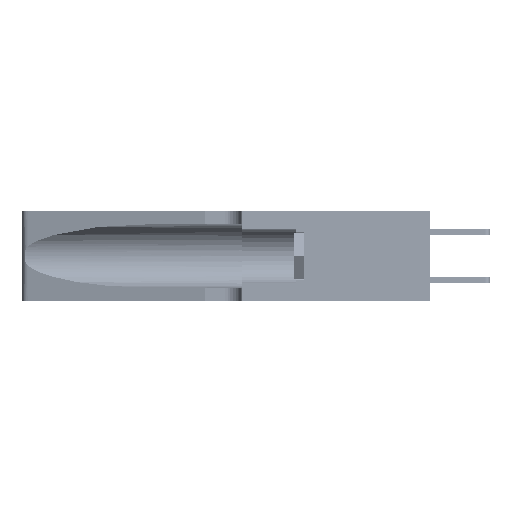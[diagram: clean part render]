
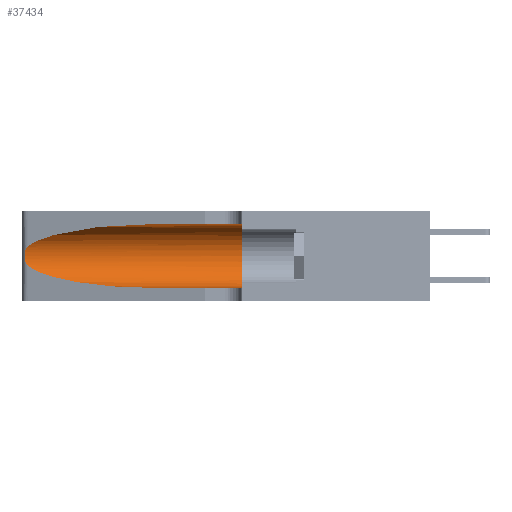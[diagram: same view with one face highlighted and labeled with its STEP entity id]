
A CAD part, left-side view. The second image highlights one B-rep face of the part: STEP entity #37434.
In plain terms, the highlighted cylindrical face has radius 3.308 mm (diameter 6.617 mm), a partial arc.
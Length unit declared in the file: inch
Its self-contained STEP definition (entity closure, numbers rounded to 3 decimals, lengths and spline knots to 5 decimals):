
#16 = ORIENTED_EDGE ( 'NONE', *, *, #25882, .T. ) ;
#394 = CARTESIAN_POINT ( 'NONE',  ( 0.26018, 1.23835, 0.19895 ) ) ;
#537 = CARTESIAN_POINT ( 'NONE',  ( 0.26017, 1.23833, 0.17102 ) ) ;
#4063 = CARTESIAN_POINT ( 'NONE',  ( 0.26075, 1.23896, 0.19203 ) ) ;
#4191 = CARTESIAN_POINT ( 'NONE',  ( 0.25856, 1.23593, 0.16098 ) ) ;
#4660 = DIRECTION ( 'NONE',  ( 0., -1., 0. ) ) ;
#5260 = FACE_OUTER_BOUND ( 'NONE', #7107, .T. ) ;
#5830 = LINE ( 'NONE', #11191, #22958 ) ;
#7107 = EDGE_LOOP ( 'NONE', ( #22844, #28178, #16, #17809, #18343, #36347 ) ) ;
#7213 = EDGE_CURVE ( 'NONE', #29267, #22690, #15760, .T. ) ;
#7237 = CARTESIAN_POINT ( 'NONE',  ( 0.25487, 1.22718, 0.14631 ) ) ;
#7265 = CYLINDRICAL_SURFACE ( 'NONE', #29936, 0.13025 ) ;
#7520 = CARTESIAN_POINT ( 'NONE',  ( 0.25787, 1.23484, 0.2124 ) ) ;
#7990 = CARTESIAN_POINT ( 'NONE',  ( 0.1305, 1.61858, 0.185 ) ) ;
#8094 = CARTESIAN_POINT ( 'NONE',  ( 0.1305, 0.72297, 0.05475 ) ) ;
#8631 = EDGE_CURVE ( 'NONE', #36880, #33583, #22777, .T. ) ;
#8737 = DIRECTION ( 'NONE',  ( 0., 0., 1. ) ) ;
#9618 = VECTOR ( 'NONE', #12274, 39.37008 ) ;
#11191 = CARTESIAN_POINT ( 'NONE',  ( 0.1305, 1.61858, 0.05475 ) ) ;
#11866 = VERTEX_POINT ( 'NONE', #37948 ) ;
#12274 = DIRECTION ( 'NONE',  ( 0., -1., 0. ) ) ;
#13554 = CARTESIAN_POINT ( 'NONE',  ( 0.1305, 0.35, 0.05475 ) ) ;
#15760 =( BOUNDED_CURVE ( )  B_SPLINE_CURVE ( 3, ( #37120, #20581, #34031, #32048 ),
 .UNSPECIFIED., .F., .F. ) 
 B_SPLINE_CURVE_WITH_KNOTS ( ( 4, 4 ),
 ( 1.5708, 2.84003 ),
 .UNSPECIFIED. ) 
 CURVE ( )  GEOMETRIC_REPRESENTATION_ITEM ( )  RATIONAL_B_SPLINE_CURVE ( ( 1., 0.87, 0.87, 1. ) ) 
 REPRESENTATION_ITEM ( '' )  );
#17014 = B_SPLINE_CURVE_WITH_KNOTS ( 'NONE', 3,
 ( #24036, #36865, #20741, #7520, #37137, #394, #4063, #20328, #537, #4191, #27388, #30696, #40222, #7237 ),
 .UNSPECIFIED., .F., .F.,
 ( 4, 2, 2, 2, 2, 2, 4 ),
 ( 0., 0.00027, 0.00053, 0.00107, 0.0016, 0.00187, 0.00214 ),
 .UNSPECIFIED. ) ;
#17809 = ORIENTED_EDGE ( 'NONE', *, *, #36655, .T. ) ;
#18343 = ORIENTED_EDGE ( 'NONE', *, *, #8631, .F. ) ;
#18480 = LINE ( 'NONE', #41313, #9618 ) ;
#18519 = CARTESIAN_POINT ( 'NONE',  ( 0.18966, 0.96281, 0.05475 ) ) ;
#20328 = CARTESIAN_POINT ( 'NONE',  ( 0.26075, 1.23896, 0.178 ) ) ;
#20581 = CARTESIAN_POINT ( 'NONE',  ( 0.18966, 0.96281, 0.31525 ) ) ;
#20741 = CARTESIAN_POINT ( 'NONE',  ( 0.25639, 1.23184, 0.21858 ) ) ;
#22690 = VERTEX_POINT ( 'NONE', #22950 ) ;
#22777 = CIRCLE ( 'NONE', #38520, 0.13025 ) ;
#22844 = ORIENTED_EDGE ( 'NONE', *, *, #7213, .T. ) ;
#22950 = CARTESIAN_POINT ( 'NONE',  ( 0.25487, 1.22718, 0.22369 ) ) ;
#22958 = VECTOR ( 'NONE', #37453, 39.37008 ) ;
#24036 = CARTESIAN_POINT ( 'NONE',  ( 0.25487, 1.22718, 0.22369 ) ) ;
#24542 = EDGE_CURVE ( 'NONE', #29267, #36880, #18480, .T. ) ;
#25009 = CARTESIAN_POINT ( 'NONE',  ( 0.25487, 1.22718, 0.14631 ) ) ;
#25882 = EDGE_CURVE ( 'NONE', #11866, #40170, #34293, .T. ) ;
#27388 = CARTESIAN_POINT ( 'NONE',  ( 0.25789, 1.23486, 0.15765 ) ) ;
#28178 = ORIENTED_EDGE ( 'NONE', *, *, #28839, .T. ) ;
#28839 = EDGE_CURVE ( 'NONE', #22690, #11866, #17014, .T. ) ;
#29267 = VERTEX_POINT ( 'NONE', #42829 ) ;
#29936 = AXIS2_PLACEMENT_3D ( 'NONE', #7990, #4660, #31158 ) ;
#30696 = CARTESIAN_POINT ( 'NONE',  ( 0.25639, 1.23186, 0.15144 ) ) ;
#31158 = DIRECTION ( 'NONE',  ( 0., 0., -1. ) ) ;
#31772 = DIRECTION ( 'NONE',  ( 0., 1., 0. ) ) ;
#32048 = CARTESIAN_POINT ( 'NONE',  ( 0.25487, 1.22718, 0.22369 ) ) ;
#32065 = CARTESIAN_POINT ( 'NONE',  ( 0.1305, 0.35, 0.185 ) ) ;
#33583 = VERTEX_POINT ( 'NONE', #13554 ) ;
#34031 = CARTESIAN_POINT ( 'NONE',  ( 0.2373, 1.15595, 0.28018 ) ) ;
#34293 =( BOUNDED_CURVE ( )  B_SPLINE_CURVE ( 3, ( #25009, #38418, #18519, #41766 ),
 .UNSPECIFIED., .F., .T. ) 
 B_SPLINE_CURVE_WITH_KNOTS ( ( 4, 4 ),
 ( 3.44316, 4.71239 ),
 .UNSPECIFIED. ) 
 CURVE ( )  GEOMETRIC_REPRESENTATION_ITEM ( )  RATIONAL_B_SPLINE_CURVE ( ( 1., 0.87, 0.87, 1. ) ) 
 REPRESENTATION_ITEM ( '' )  );
#35744 = CARTESIAN_POINT ( 'NONE',  ( 0.1305, 0.35, 0.31525 ) ) ;
#36347 = ORIENTED_EDGE ( 'NONE', *, *, #24542, .F. ) ;
#36655 = EDGE_CURVE ( 'NONE', #40170, #33583, #5830, .T. ) ;
#36865 = CARTESIAN_POINT ( 'NONE',  ( 0.25555, 1.22994, 0.2215 ) ) ;
#36880 = VERTEX_POINT ( 'NONE', #35744 ) ;
#37120 = CARTESIAN_POINT ( 'NONE',  ( 0.1305, 0.72297, 0.31525 ) ) ;
#37137 = CARTESIAN_POINT ( 'NONE',  ( 0.25854, 1.2359, 0.20912 ) ) ;
#37434 = ADVANCED_FACE ( 'NONE', ( #5260 ), #7265, .F. ) ;
#37453 = DIRECTION ( 'NONE',  ( 0., -1., 0. ) ) ;
#37948 = CARTESIAN_POINT ( 'NONE',  ( 0.25487, 1.22718, 0.14631 ) ) ;
#38418 = CARTESIAN_POINT ( 'NONE',  ( 0.2373, 1.15595, 0.08982 ) ) ;
#38520 = AXIS2_PLACEMENT_3D ( 'NONE', #32065, #31772, #8737 ) ;
#40170 = VERTEX_POINT ( 'NONE', #8094 ) ;
#40222 = CARTESIAN_POINT ( 'NONE',  ( 0.25555, 1.22993, 0.14849 ) ) ;
#41313 = CARTESIAN_POINT ( 'NONE',  ( 0.1305, 1.61858, 0.31525 ) ) ;
#41766 = CARTESIAN_POINT ( 'NONE',  ( 0.1305, 0.72297, 0.05475 ) ) ;
#42829 = CARTESIAN_POINT ( 'NONE',  ( 0.1305, 0.72297, 0.31525 ) ) ;
